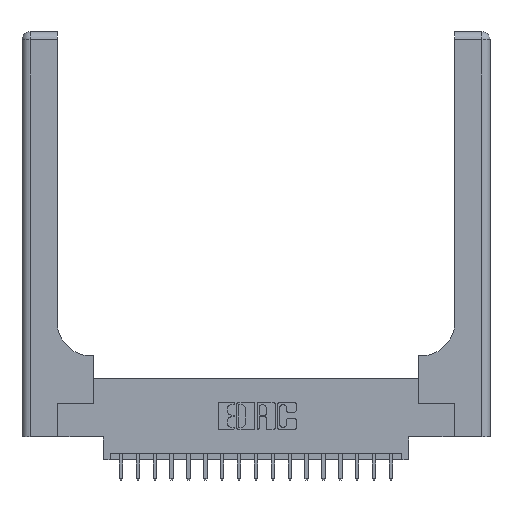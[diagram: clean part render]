
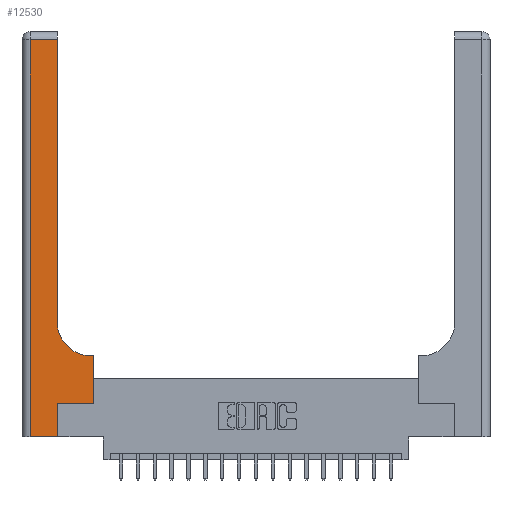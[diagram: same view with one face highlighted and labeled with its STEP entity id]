
A CAD part, top view. The second image highlights one B-rep face of the part: STEP entity #12530.
In plain terms, the highlighted planar face has unit normal (0, 0, 1).
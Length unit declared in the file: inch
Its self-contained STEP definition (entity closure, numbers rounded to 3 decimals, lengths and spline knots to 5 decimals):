
#276 = PLANE ( 'NONE',  #10572 ) ;
#467 = CARTESIAN_POINT ( 'NONE',  ( 0.06, 0., 0.37 ) ) ;
#585 = CARTESIAN_POINT ( 'NONE',  ( 0., 3., 0.37 ) ) ;
#866 = VECTOR ( 'NONE', #13369, 39.37008 ) ;
#1369 = CARTESIAN_POINT ( 'NONE',  ( 0., 2.94, 0.37 ) ) ;
#1657 = LINE ( 'NONE', #10776, #6418 ) ;
#1746 = EDGE_CURVE ( 'NONE', #10356, #3663, #12332, .T. ) ;
#2326 = DIRECTION ( 'NONE',  ( 1., 0., 0. ) ) ;
#2391 = EDGE_LOOP ( 'NONE', ( #15285, #7072, #4149, #20212, #16212, #3449, #2932, #14769, #2655 ) ) ;
#2655 = ORIENTED_EDGE ( 'NONE', *, *, #2837, .T. ) ;
#2740 = EDGE_CURVE ( 'NONE', #4499, #10356, #8577, .T. ) ;
#2837 = EDGE_CURVE ( 'NONE', #3976, #4499, #11593, .T. ) ;
#2927 = VECTOR ( 'NONE', #7207, 39.37008 ) ;
#2932 = ORIENTED_EDGE ( 'NONE', *, *, #9244, .T. ) ;
#2983 = DIRECTION ( 'NONE',  ( -1., 0., 0. ) ) ;
#3214 = VERTEX_POINT ( 'NONE', #467 ) ;
#3449 = ORIENTED_EDGE ( 'NONE', *, *, #13302, .T. ) ;
#3519 = DIRECTION ( 'NONE',  ( 0., 1., 0. ) ) ;
#3557 = DIRECTION ( 'NONE',  ( 1., 0., 0. ) ) ;
#3663 = VERTEX_POINT ( 'NONE', #19354 ) ;
#3976 = VERTEX_POINT ( 'NONE', #12705 ) ;
#4149 = ORIENTED_EDGE ( 'NONE', *, *, #14295, .T. ) ;
#4499 = VERTEX_POINT ( 'NONE', #9687 ) ;
#5040 = AXIS2_PLACEMENT_3D ( 'NONE', #13199, #16347, #2326 ) ;
#5329 = CARTESIAN_POINT ( 'NONE',  ( 0.265, 0.25, 0.37 ) ) ;
#6418 = VECTOR ( 'NONE', #2983, 39.37008 ) ;
#6536 = DIRECTION ( 'NONE',  ( -1., 0., 0. ) ) ;
#6750 = DIRECTION ( 'NONE',  ( 0., 1., 0. ) ) ;
#6828 = VECTOR ( 'NONE', #3557, 39.37008 ) ;
#7072 = ORIENTED_EDGE ( 'NONE', *, *, #1746, .T. ) ;
#7207 = DIRECTION ( 'NONE',  ( 0., 1., 0. ) ) ;
#7841 = CARTESIAN_POINT ( 'NONE',  ( 0.26, 2.94, 0.37 ) ) ;
#7992 = VECTOR ( 'NONE', #16790, 39.37008 ) ;
#8017 = VECTOR ( 'NONE', #6750, 39.37008 ) ;
#8577 = LINE ( 'NONE', #14929, #8017 ) ;
#8943 = LINE ( 'NONE', #15176, #866 ) ;
#9124 = CARTESIAN_POINT ( 'NONE',  ( 0.265, 0., 0.37 ) ) ;
#9244 = EDGE_CURVE ( 'NONE', #9421, #12997, #17824, .T. ) ;
#9421 = VERTEX_POINT ( 'NONE', #14984 ) ;
#9491 = VECTOR ( 'NONE', #10028, 39.37008 ) ;
#9597 = VECTOR ( 'NONE', #3519, 39.37008 ) ;
#9687 = CARTESIAN_POINT ( 'NONE',  ( 0.26, 0.85, 0.37 ) ) ;
#10028 = DIRECTION ( 'NONE',  ( 1., 0., 0. ) ) ;
#10223 = CARTESIAN_POINT ( 'NONE',  ( 0.265, 0.25, 0.37 ) ) ;
#10356 = VERTEX_POINT ( 'NONE', #7841 ) ;
#10572 = AXIS2_PLACEMENT_3D ( 'NONE', #585, #16037, #6536 ) ;
#10776 = CARTESIAN_POINT ( 'NONE',  ( 0.26, 0.6, 0.37 ) ) ;
#10914 = CARTESIAN_POINT ( 'NONE',  ( 0.265, 0., 0.37 ) ) ;
#11247 = FACE_OUTER_BOUND ( 'NONE', #2391, .T. ) ;
#11359 = EDGE_CURVE ( 'NONE', #19490, #16108, #16779, .T. ) ;
#11593 = CIRCLE ( 'NONE', #5040, 0.25 ) ;
#11601 = EDGE_CURVE ( 'NONE', #12997, #3976, #1657, .T. ) ;
#12332 = LINE ( 'NONE', #1369, #7992 ) ;
#12530 = ADVANCED_FACE ( 'NONE', ( #11247 ), #276, .F. ) ;
#12705 = CARTESIAN_POINT ( 'NONE',  ( 0.51, 0.6, 0.37 ) ) ;
#12997 = VERTEX_POINT ( 'NONE', #18112 ) ;
#13059 = CARTESIAN_POINT ( 'NONE',  ( 0.528, 0.25, 0.37 ) ) ;
#13199 = CARTESIAN_POINT ( 'NONE',  ( 0.51, 0.85, 0.37 ) ) ;
#13302 = EDGE_CURVE ( 'NONE', #16108, #9421, #19343, .T. ) ;
#13369 = DIRECTION ( 'NONE',  ( 0., -1., 0. ) ) ;
#13744 = EDGE_CURVE ( 'NONE', #3214, #19490, #19321, .T. ) ;
#14295 = EDGE_CURVE ( 'NONE', #3663, #3214, #8943, .T. ) ;
#14769 = ORIENTED_EDGE ( 'NONE', *, *, #11601, .T. ) ;
#14929 = CARTESIAN_POINT ( 'NONE',  ( 0.26, 3., 0.37 ) ) ;
#14984 = CARTESIAN_POINT ( 'NONE',  ( 0.528, 0.25, 0.37 ) ) ;
#15176 = CARTESIAN_POINT ( 'NONE',  ( 0.06, 3., 0.37 ) ) ;
#15285 = ORIENTED_EDGE ( 'NONE', *, *, #2740, .T. ) ;
#16037 = DIRECTION ( 'NONE',  ( 0., 0., -1. ) ) ;
#16108 = VERTEX_POINT ( 'NONE', #10223 ) ;
#16212 = ORIENTED_EDGE ( 'NONE', *, *, #11359, .T. ) ;
#16235 = CARTESIAN_POINT ( 'NONE',  ( 0., 0., 0.37 ) ) ;
#16347 = DIRECTION ( 'NONE',  ( 0., 0., -1. ) ) ;
#16779 = LINE ( 'NONE', #9124, #2927 ) ;
#16790 = DIRECTION ( 'NONE',  ( -1., 0., 0. ) ) ;
#17824 = LINE ( 'NONE', #13059, #9597 ) ;
#18112 = CARTESIAN_POINT ( 'NONE',  ( 0.528, 0.6, 0.37 ) ) ;
#19321 = LINE ( 'NONE', #16235, #6828 ) ;
#19343 = LINE ( 'NONE', #5329, #9491 ) ;
#19354 = CARTESIAN_POINT ( 'NONE',  ( 0.06, 2.94, 0.37 ) ) ;
#19490 = VERTEX_POINT ( 'NONE', #10914 ) ;
#20212 = ORIENTED_EDGE ( 'NONE', *, *, #13744, .T. ) ;
